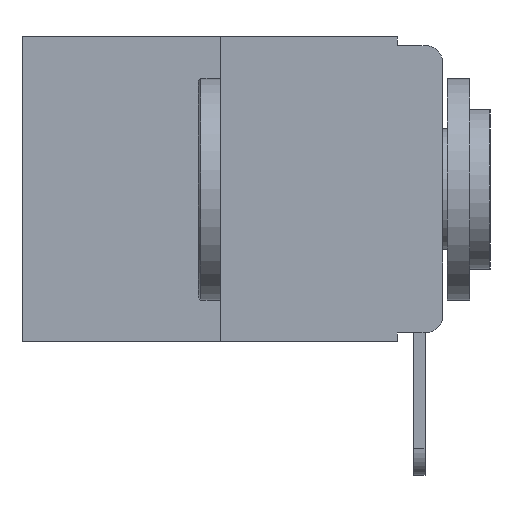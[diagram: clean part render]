
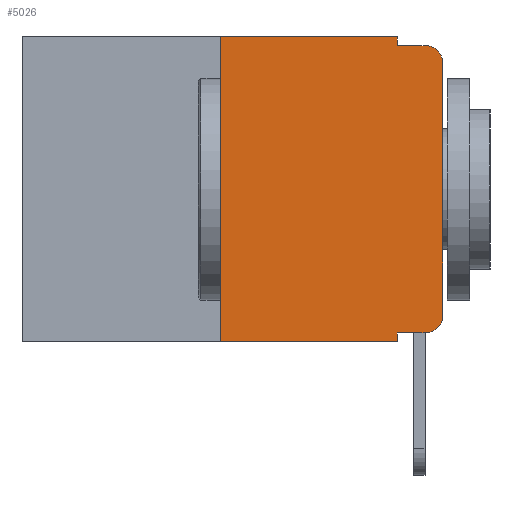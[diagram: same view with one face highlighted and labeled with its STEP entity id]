
A CAD part, left-side view. The second image highlights one B-rep face of the part: STEP entity #5026.
In plain terms, the highlighted planar face has unit normal (-1, 0, 0).
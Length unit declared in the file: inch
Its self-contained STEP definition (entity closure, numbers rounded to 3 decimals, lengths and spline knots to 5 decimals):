
#412 = EDGE_CURVE ( 'NONE', #7019, #11255, #3876, .T. ) ;
#605 = EDGE_CURVE ( 'NONE', #18023, #10777, #2580, .T. ) ;
#767 = CARTESIAN_POINT ( 'NONE',  ( 0., 0.02, -0.333 ) ) ;
#808 = CARTESIAN_POINT ( 'NONE',  ( 0., 0., 0. ) ) ;
#1121 = DIRECTION ( 'NONE',  ( 0., -1., 0. ) ) ;
#1876 = ORIENTED_EDGE ( 'NONE', *, *, #5742, .T. ) ;
#1880 = ORIENTED_EDGE ( 'NONE', *, *, #412, .T. ) ;
#2202 = CARTESIAN_POINT ( 'NONE',  ( 0., 0.02, -0.03 ) ) ;
#2580 = LINE ( 'NONE', #6274, #13039 ) ;
#2748 = DIRECTION ( 'NONE',  ( 0., 0., -1. ) ) ;
#2905 = LINE ( 'NONE', #6401, #13111 ) ;
#3021 = VERTEX_POINT ( 'NONE', #15645 ) ;
#3048 = DIRECTION ( 'NONE',  ( 0., 0., -1. ) ) ;
#3122 = EDGE_LOOP ( 'NONE', ( #5863, #1880, #15649, #7568, #8832, #20690, #1876, #14837, #4324, #6760 ) ) ;
#3327 = LINE ( 'NONE', #808, #11989 ) ;
#3870 = DIRECTION ( 'NONE',  ( -1., 0., 0. ) ) ;
#3876 = CIRCLE ( 'NONE', #9620, 0.02 ) ;
#3878 = VERTEX_POINT ( 'NONE', #8515 ) ;
#3953 = VERTEX_POINT ( 'NONE', #7099 ) ;
#3960 = EDGE_CURVE ( 'NONE', #10777, #4981, #8314, .T. ) ;
#4010 = DIRECTION ( 'NONE',  ( 0., -1., 0. ) ) ;
#4181 = CARTESIAN_POINT ( 'NONE',  ( 0., 0.473, -0.343 ) ) ;
#4324 = ORIENTED_EDGE ( 'NONE', *, *, #605, .T. ) ;
#4981 = VERTEX_POINT ( 'NONE', #8407 ) ;
#5026 = ADVANCED_FACE ( 'NONE', ( #12994 ), #10501, .F. ) ;
#5500 = DIRECTION ( 'NONE',  ( 0., 0., 1. ) ) ;
#5742 = EDGE_CURVE ( 'NONE', #3953, #8996, #8366, .T. ) ;
#5781 = DIRECTION ( 'NONE',  ( 1., 0., 0. ) ) ;
#5852 = CARTESIAN_POINT ( 'NONE',  ( 0., 0.473, 0. ) ) ;
#5863 = ORIENTED_EDGE ( 'NONE', *, *, #16398, .T. ) ;
#6076 = CARTESIAN_POINT ( 'NONE',  ( 0., 0., -0.03 ) ) ;
#6274 = CARTESIAN_POINT ( 'NONE',  ( 0., 0.051, -0.333 ) ) ;
#6369 = VECTOR ( 'NONE', #2748, 39.37008 ) ;
#6401 = CARTESIAN_POINT ( 'NONE',  ( 0., 0.051, 0. ) ) ;
#6450 = EDGE_CURVE ( 'NONE', #3953, #3878, #14996, .T. ) ;
#6465 = DIRECTION ( 'NONE',  ( 0., -1., 0. ) ) ;
#6760 = ORIENTED_EDGE ( 'NONE', *, *, #3960, .T. ) ;
#6806 = VECTOR ( 'NONE', #4010, 39.37008 ) ;
#6914 = EDGE_CURVE ( 'NONE', #3878, #19164, #11645, .T. ) ;
#7019 = VERTEX_POINT ( 'NONE', #6076 ) ;
#7099 = CARTESIAN_POINT ( 'NONE',  ( 0., 0.25, -0.343 ) ) ;
#7377 = DIRECTION ( 'NONE',  ( 0., 0., 1. ) ) ;
#7568 = ORIENTED_EDGE ( 'NONE', *, *, #14262, .F. ) ;
#8168 = LINE ( 'NONE', #15804, #6369 ) ;
#8314 = CIRCLE ( 'NONE', #13923, 0.02 ) ;
#8366 = LINE ( 'NONE', #4181, #10393 ) ;
#8407 = CARTESIAN_POINT ( 'NONE',  ( 0., 0., -0.313 ) ) ;
#8515 = CARTESIAN_POINT ( 'NONE',  ( 0., 0.25, 0. ) ) ;
#8832 = ORIENTED_EDGE ( 'NONE', *, *, #6914, .F. ) ;
#8996 = VERTEX_POINT ( 'NONE', #12730 ) ;
#9010 = DIRECTION ( 'NONE',  ( 0., 0., -1. ) ) ;
#9620 = AXIS2_PLACEMENT_3D ( 'NONE', #2202, #3870, #13412 ) ;
#10393 = VECTOR ( 'NONE', #20275, 39.37008 ) ;
#10423 = DIRECTION ( 'NONE',  ( 0., 0., -1. ) ) ;
#10501 = PLANE ( 'NONE',  #12588 ) ;
#10777 = VERTEX_POINT ( 'NONE', #767 ) ;
#11255 = VERTEX_POINT ( 'NONE', #13823 ) ;
#11645 = LINE ( 'NONE', #15332, #6806 ) ;
#11989 = VECTOR ( 'NONE', #5500, 39.37008 ) ;
#12588 = AXIS2_PLACEMENT_3D ( 'NONE', #5852, #5781, #9010 ) ;
#12693 = CARTESIAN_POINT ( 'NONE',  ( 0., 0.051, -0.333 ) ) ;
#12730 = CARTESIAN_POINT ( 'NONE',  ( 0., 0.051, -0.343 ) ) ;
#12994 = FACE_OUTER_BOUND ( 'NONE', #3122, .T. ) ;
#13039 = VECTOR ( 'NONE', #1121, 39.37008 ) ;
#13111 = VECTOR ( 'NONE', #3048, 39.37008 ) ;
#13412 = DIRECTION ( 'NONE',  ( 0., 0., -1. ) ) ;
#13823 = CARTESIAN_POINT ( 'NONE',  ( 0., 0.02, -0.01 ) ) ;
#13923 = AXIS2_PLACEMENT_3D ( 'NONE', #15844, #16931, #10423 ) ;
#14262 = EDGE_CURVE ( 'NONE', #19164, #3021, #2905, .T. ) ;
#14805 = VECTOR ( 'NONE', #6465, 39.37008 ) ;
#14837 = ORIENTED_EDGE ( 'NONE', *, *, #16586, .F. ) ;
#14996 = LINE ( 'NONE', #15498, #19070 ) ;
#15332 = CARTESIAN_POINT ( 'NONE',  ( 0., 0.473, 0. ) ) ;
#15498 = CARTESIAN_POINT ( 'NONE',  ( 0., 0.25, 0. ) ) ;
#15645 = CARTESIAN_POINT ( 'NONE',  ( 0., 0.051, -0.01 ) ) ;
#15649 = ORIENTED_EDGE ( 'NONE', *, *, #18634, .F. ) ;
#15804 = CARTESIAN_POINT ( 'NONE',  ( 0., 0.051, 0. ) ) ;
#15844 = CARTESIAN_POINT ( 'NONE',  ( 0., 0.02, -0.313 ) ) ;
#16398 = EDGE_CURVE ( 'NONE', #4981, #7019, #3327, .T. ) ;
#16586 = EDGE_CURVE ( 'NONE', #18023, #8996, #8168, .T. ) ;
#16931 = DIRECTION ( 'NONE',  ( -1., 0., 0. ) ) ;
#17080 = LINE ( 'NONE', #21011, #14805 ) ;
#18023 = VERTEX_POINT ( 'NONE', #12693 ) ;
#18634 = EDGE_CURVE ( 'NONE', #3021, #11255, #17080, .T. ) ;
#19070 = VECTOR ( 'NONE', #7377, 39.37008 ) ;
#19164 = VERTEX_POINT ( 'NONE', #20776 ) ;
#20275 = DIRECTION ( 'NONE',  ( 0., -1., 0. ) ) ;
#20690 = ORIENTED_EDGE ( 'NONE', *, *, #6450, .F. ) ;
#20776 = CARTESIAN_POINT ( 'NONE',  ( 0., 0.051, 0. ) ) ;
#21011 = CARTESIAN_POINT ( 'NONE',  ( 0., 0.051, -0.01 ) ) ;
